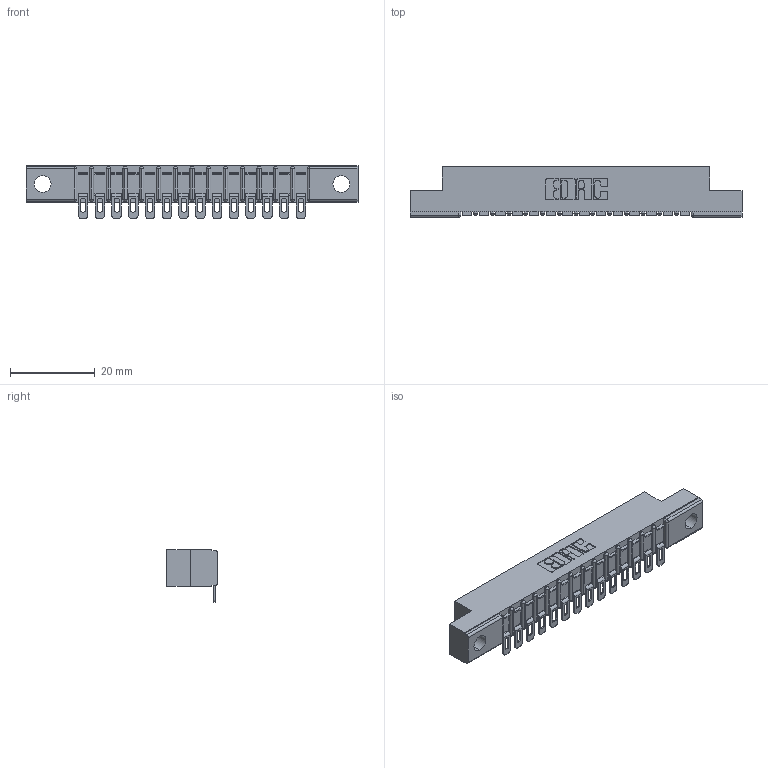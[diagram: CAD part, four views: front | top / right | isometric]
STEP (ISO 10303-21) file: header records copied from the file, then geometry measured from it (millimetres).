
FILE_DESCRIPTION (( 'STEP AP203' ), '1' );
FILE_NAME ('357-014-454-104.STEP', '2020-09-30T16:23:36', ( '' ), ( '' ), 'SwSTEP 2.0', 'SolidWorks 2020', '' );
FILE_SCHEMA (( 'CONFIG_CONTROL_DESIGN' ));
Length unit declared in the file: inch
Products named in the file (3): 307 Part_.156 Dia Mounting Holes; 307-290-002_554; 357-014-454-104
Assembly tree (15 placements, depth 2):
  357-014-454-104
    307 Part_.156 Dia Mounting Holes
    307-290-002_554  x14
Bounding box: 78.49 x 12.01 x 12.52 mm (x, y, z)
Volume: 5076.4 mm3; surface area: 8736.7 mm2
Topology: 15 solids, 15 shells, 1281 faces, 3901 edges, 2558 vertices
Faces by surface type: plane 728, cylinder 523, sphere 30
Entity records: 16837 total; most frequent: CARTESIAN_POINT 2840, ORIENTED_EDGE 2828, DIRECTION 2770, EDGE_CURVE 1414, VECTOR 1070, LINE 1070, VERTEX_POINT 920, AXIS2_PLACEMENT_3D 850
